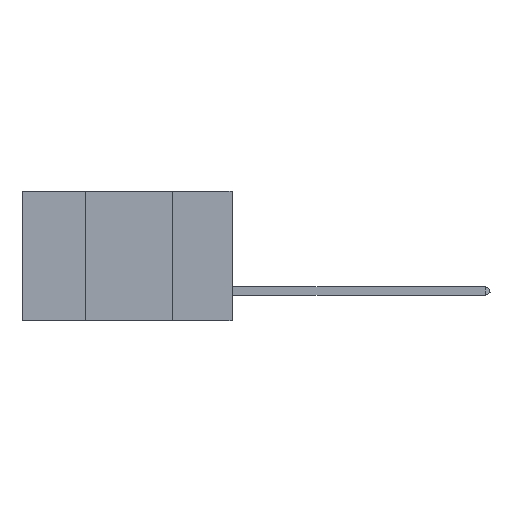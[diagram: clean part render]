
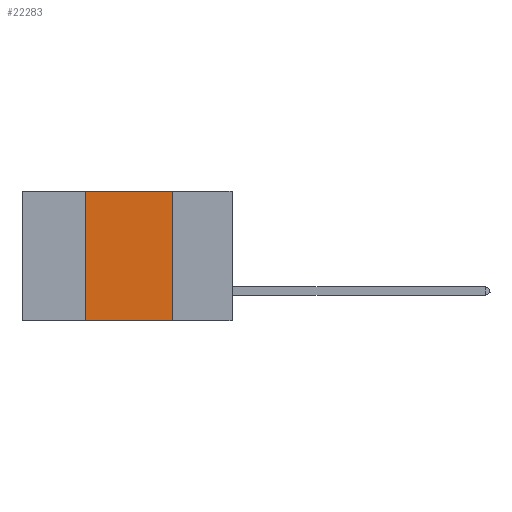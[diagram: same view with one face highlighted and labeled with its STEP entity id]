
A CAD part, left-side view. The second image highlights one B-rep face of the part: STEP entity #22283.
In plain terms, the highlighted planar face has unit normal (-1, 0, 0).
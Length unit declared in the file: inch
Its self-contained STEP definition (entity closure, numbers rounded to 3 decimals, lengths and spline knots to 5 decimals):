
#132 = DIRECTION ( 'NONE',  ( 0., -1., 0. ) ) ;
#248 = ORIENTED_EDGE ( 'NONE', *, *, #16472, .T. ) ;
#277 = CARTESIAN_POINT ( 'NONE',  ( 0., 0.42, -0.37 ) ) ;
#594 = LINE ( 'NONE', #15239, #21938 ) ;
#2941 = EDGE_LOOP ( 'NONE', ( #21108, #6167, #20626, #248 ) ) ;
#3001 = CARTESIAN_POINT ( 'NONE',  ( 0., 0.17, 0. ) ) ;
#4029 = EDGE_CURVE ( 'NONE', #17580, #21436, #594, .T. ) ;
#4998 = LINE ( 'NONE', #6070, #19476 ) ;
#5409 = VERTEX_POINT ( 'NONE', #23448 ) ;
#5831 = DIRECTION ( 'NONE',  ( 1., 0., 0. ) ) ;
#6070 = CARTESIAN_POINT ( 'NONE',  ( 0., 0.42, 0. ) ) ;
#6167 = ORIENTED_EDGE ( 'NONE', *, *, #4029, .F. ) ;
#6417 = DIRECTION ( 'NONE',  ( 0., 0., 1. ) ) ;
#8032 = AXIS2_PLACEMENT_3D ( 'NONE', #13655, #5831, #26026 ) ;
#9457 = CARTESIAN_POINT ( 'NONE',  ( 0., 0.6, -0.37 ) ) ;
#10843 = EDGE_CURVE ( 'NONE', #20881, #17580, #4998, .T. ) ;
#11264 = FACE_OUTER_BOUND ( 'NONE', #2941, .T. ) ;
#12394 = LINE ( 'NONE', #3001, #21764 ) ;
#13655 = CARTESIAN_POINT ( 'NONE',  ( 0., 0.6, 0. ) ) ;
#15239 = CARTESIAN_POINT ( 'NONE',  ( 0., 0.6, 0. ) ) ;
#16077 = PLANE ( 'NONE',  #8032 ) ;
#16472 = EDGE_CURVE ( 'NONE', #20881, #5409, #22564, .T. ) ;
#17051 = VECTOR ( 'NONE', #132, 39.37008 ) ;
#17415 = DIRECTION ( 'NONE',  ( 0., 0., -1. ) ) ;
#17580 = VERTEX_POINT ( 'NONE', #25923 ) ;
#17629 = CARTESIAN_POINT ( 'NONE',  ( 0., 0.17, 0. ) ) ;
#19476 = VECTOR ( 'NONE', #6417, 39.37008 ) ;
#20626 = ORIENTED_EDGE ( 'NONE', *, *, #10843, .F. ) ;
#20881 = VERTEX_POINT ( 'NONE', #277 ) ;
#21108 = ORIENTED_EDGE ( 'NONE', *, *, #25137, .F. ) ;
#21436 = VERTEX_POINT ( 'NONE', #17629 ) ;
#21764 = VECTOR ( 'NONE', #17415, 39.37008 ) ;
#21938 = VECTOR ( 'NONE', #25527, 39.37008 ) ;
#22283 = ADVANCED_FACE ( 'NONE', ( #11264 ), #16077, .F. ) ;
#22564 = LINE ( 'NONE', #9457, #17051 ) ;
#23448 = CARTESIAN_POINT ( 'NONE',  ( 0., 0.17, -0.37 ) ) ;
#25137 = EDGE_CURVE ( 'NONE', #21436, #5409, #12394, .T. ) ;
#25527 = DIRECTION ( 'NONE',  ( 0., -1., 0. ) ) ;
#25923 = CARTESIAN_POINT ( 'NONE',  ( 0., 0.42, 0. ) ) ;
#26026 = DIRECTION ( 'NONE',  ( 0., 0., -1. ) ) ;
